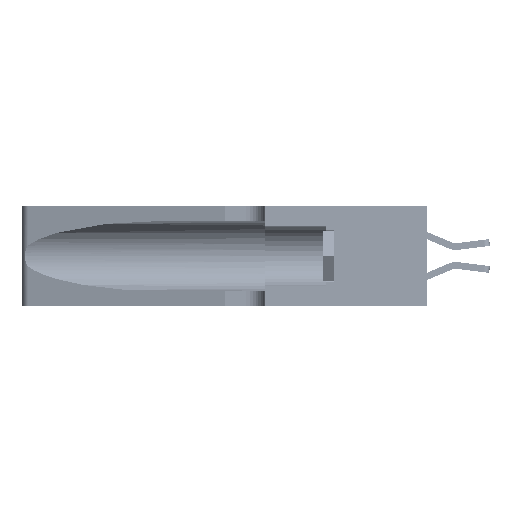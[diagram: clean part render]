
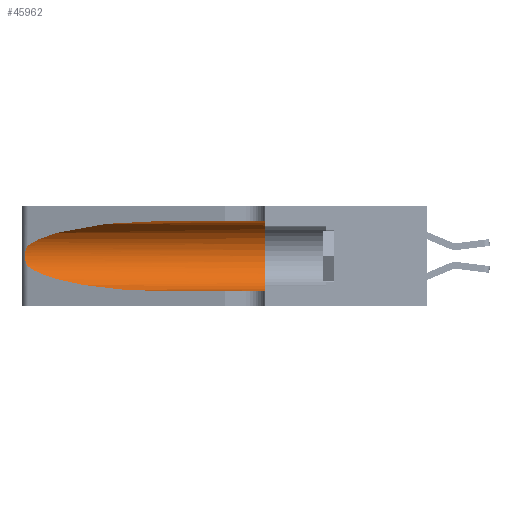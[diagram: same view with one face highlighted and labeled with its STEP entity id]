
A CAD part, left-side view. The second image highlights one B-rep face of the part: STEP entity #45962.
In plain terms, the highlighted cylindrical face has radius 3.308 mm (diameter 6.617 mm), a partial arc.
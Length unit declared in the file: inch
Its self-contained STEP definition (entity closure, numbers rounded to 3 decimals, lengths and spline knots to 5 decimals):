
#1337 = CARTESIAN_POINT ( 'NONE',  ( 0.1305, 1.61858, 0.05475 ) ) ;
#1681 = CARTESIAN_POINT ( 'NONE',  ( 0.25787, 1.23484, 0.2124 ) ) ;
#1777 = CARTESIAN_POINT ( 'NONE',  ( 0.1305, 0.72297, 0.05475 ) ) ;
#1945 = VERTEX_POINT ( 'NONE', #23181 ) ;
#2078 = CARTESIAN_POINT ( 'NONE',  ( 0.18966, 0.96281, 0.05475 ) ) ;
#2089 = VECTOR ( 'NONE', #41808, 39.37008 ) ;
#2421 = CARTESIAN_POINT ( 'NONE',  ( 0.25487, 1.22718, 0.22369 ) ) ;
#2812 =( BOUNDED_CURVE ( )  B_SPLINE_CURVE ( 3, ( #40480, #14954, #44198, #22348 ),
 .UNSPECIFIED., .F., .T. ) 
 B_SPLINE_CURVE_WITH_KNOTS ( ( 4, 4 ),
 ( 1.5708, 2.84003 ),
 .UNSPECIFIED. ) 
 CURVE ( )  GEOMETRIC_REPRESENTATION_ITEM ( )  RATIONAL_B_SPLINE_CURVE ( ( 1., 0.87, 0.87, 1. ) ) 
 REPRESENTATION_ITEM ( '' )  );
#2910 = AXIS2_PLACEMENT_3D ( 'NONE', #28541, #6415, #32216 ) ;
#4969 = VERTEX_POINT ( 'NONE', #11466 ) ;
#5225 = CARTESIAN_POINT ( 'NONE',  ( 0.1305, 1.61858, 0.185 ) ) ;
#5509 = CARTESIAN_POINT ( 'NONE',  ( 0.26018, 1.23835, 0.19895 ) ) ;
#6415 = DIRECTION ( 'NONE',  ( 0., 1., 0. ) ) ;
#6981 = CYLINDRICAL_SURFACE ( 'NONE', #27076, 0.13025 ) ;
#8419 = VERTEX_POINT ( 'NONE', #11199 ) ;
#8901 = ORIENTED_EDGE ( 'NONE', *, *, #42480, .T. ) ;
#8976 = DIRECTION ( 'NONE',  ( 0., 0., -1. ) ) ;
#9090 = EDGE_CURVE ( 'NONE', #8419, #13979, #2812, .T. ) ;
#9248 = CARTESIAN_POINT ( 'NONE',  ( 0.26075, 1.23896, 0.178 ) ) ;
#11199 = CARTESIAN_POINT ( 'NONE',  ( 0.1305, 0.72297, 0.31525 ) ) ;
#11466 = CARTESIAN_POINT ( 'NONE',  ( 0.25487, 1.22718, 0.14631 ) ) ;
#12013 = VERTEX_POINT ( 'NONE', #47158 ) ;
#12623 = CARTESIAN_POINT ( 'NONE',  ( 0.1305, 1.61858, 0.31525 ) ) ;
#13019 = CARTESIAN_POINT ( 'NONE',  ( 0.25856, 1.23593, 0.16098 ) ) ;
#13686 = ORIENTED_EDGE ( 'NONE', *, *, #36476, .T. ) ;
#13979 = VERTEX_POINT ( 'NONE', #2421 ) ;
#14954 = CARTESIAN_POINT ( 'NONE',  ( 0.18966, 0.96281, 0.31525 ) ) ;
#16390 = DIRECTION ( 'NONE',  ( 0., -1., 0. ) ) ;
#16523 = DIRECTION ( 'NONE',  ( 0., -1., 0. ) ) ;
#16640 = CARTESIAN_POINT ( 'NONE',  ( 0.25555, 1.22994, 0.2215 ) ) ;
#16792 = CARTESIAN_POINT ( 'NONE',  ( 0.25639, 1.23186, 0.15144 ) ) ;
#20294 = CARTESIAN_POINT ( 'NONE',  ( 0.25487, 1.22718, 0.22369 ) ) ;
#20441 = CARTESIAN_POINT ( 'NONE',  ( 0.25487, 1.22718, 0.14631 ) ) ;
#20682 = CARTESIAN_POINT ( 'NONE',  ( 0.25487, 1.22718, 0.14631 ) ) ;
#20826 = VECTOR ( 'NONE', #16390, 39.37008 ) ;
#22348 = CARTESIAN_POINT ( 'NONE',  ( 0.25487, 1.22718, 0.22369 ) ) ;
#23181 = CARTESIAN_POINT ( 'NONE',  ( 0.1305, 0.35, 0.31525 ) ) ;
#24001 = CARTESIAN_POINT ( 'NONE',  ( 0.25639, 1.23184, 0.21858 ) ) ;
#24619 = EDGE_CURVE ( 'NONE', #1945, #12013, #35994, .T. ) ;
#27076 = AXIS2_PLACEMENT_3D ( 'NONE', #5225, #16523, #8976 ) ;
#27559 = EDGE_CURVE ( 'NONE', #13979, #4969, #30153, .T. ) ;
#27665 = CARTESIAN_POINT ( 'NONE',  ( 0.25854, 1.2359, 0.20912 ) ) ;
#28047 = CARTESIAN_POINT ( 'NONE',  ( 0.1305, 0.72297, 0.05475 ) ) ;
#28541 = CARTESIAN_POINT ( 'NONE',  ( 0.1305, 0.35, 0.185 ) ) ;
#30153 = B_SPLINE_CURVE_WITH_KNOTS ( 'NONE', 3,
 ( #20294, #16640, #24001, #1681, #27665, #5509, #31342, #9248, #35010, #13019, #38664, #16792, #42322, #20441 ),
 .UNSPECIFIED., .F., .F.,
 ( 4, 2, 2, 2, 2, 2, 4 ),
 ( 0., 0.00027, 0.00053, 0.00107, 0.0016, 0.00187, 0.00214 ),
 .UNSPECIFIED. ) ;
#31342 = CARTESIAN_POINT ( 'NONE',  ( 0.26075, 1.23896, 0.19203 ) ) ;
#32216 = DIRECTION ( 'NONE',  ( 0., 0., 1. ) ) ;
#32279 = VERTEX_POINT ( 'NONE', #1777 ) ;
#32787 = LINE ( 'NONE', #1337, #2089 ) ;
#33893 = ORIENTED_EDGE ( 'NONE', *, *, #24619, .F. ) ;
#35010 = CARTESIAN_POINT ( 'NONE',  ( 0.26017, 1.23833, 0.17102 ) ) ;
#35994 = CIRCLE ( 'NONE', #2910, 0.13025 ) ;
#36353 = FACE_OUTER_BOUND ( 'NONE', #40645, .T. ) ;
#36476 = EDGE_CURVE ( 'NONE', #32279, #12013, #32787, .T. ) ;
#37589 = ORIENTED_EDGE ( 'NONE', *, *, #9090, .T. ) ;
#37987 = ORIENTED_EDGE ( 'NONE', *, *, #27559, .T. ) ;
#38058 = ORIENTED_EDGE ( 'NONE', *, *, #46981, .F. ) ;
#38664 = CARTESIAN_POINT ( 'NONE',  ( 0.25789, 1.23486, 0.15765 ) ) ;
#39099 = LINE ( 'NONE', #12623, #20826 ) ;
#40480 = CARTESIAN_POINT ( 'NONE',  ( 0.1305, 0.72297, 0.31525 ) ) ;
#40645 = EDGE_LOOP ( 'NONE', ( #37589, #37987, #8901, #13686, #33893, #38058 ) ) ;
#41808 = DIRECTION ( 'NONE',  ( 0., -1., 0. ) ) ;
#42322 = CARTESIAN_POINT ( 'NONE',  ( 0.25555, 1.22993, 0.14849 ) ) ;
#42480 = EDGE_CURVE ( 'NONE', #4969, #32279, #43566, .T. ) ;
#42547 = CARTESIAN_POINT ( 'NONE',  ( 0.2373, 1.15595, 0.08982 ) ) ;
#43566 =( BOUNDED_CURVE ( )  B_SPLINE_CURVE ( 3, ( #20682, #42547, #2078, #28047 ),
 .UNSPECIFIED., .F., .F. ) 
 B_SPLINE_CURVE_WITH_KNOTS ( ( 4, 4 ),
 ( 3.44316, 4.71239 ),
 .UNSPECIFIED. ) 
 CURVE ( )  GEOMETRIC_REPRESENTATION_ITEM ( )  RATIONAL_B_SPLINE_CURVE ( ( 1., 0.87, 0.87, 1. ) ) 
 REPRESENTATION_ITEM ( '' )  );
#44198 = CARTESIAN_POINT ( 'NONE',  ( 0.2373, 1.15595, 0.28018 ) ) ;
#45962 = ADVANCED_FACE ( 'NONE', ( #36353 ), #6981, .F. ) ;
#46981 = EDGE_CURVE ( 'NONE', #8419, #1945, #39099, .T. ) ;
#47158 = CARTESIAN_POINT ( 'NONE',  ( 0.1305, 0.35, 0.05475 ) ) ;
